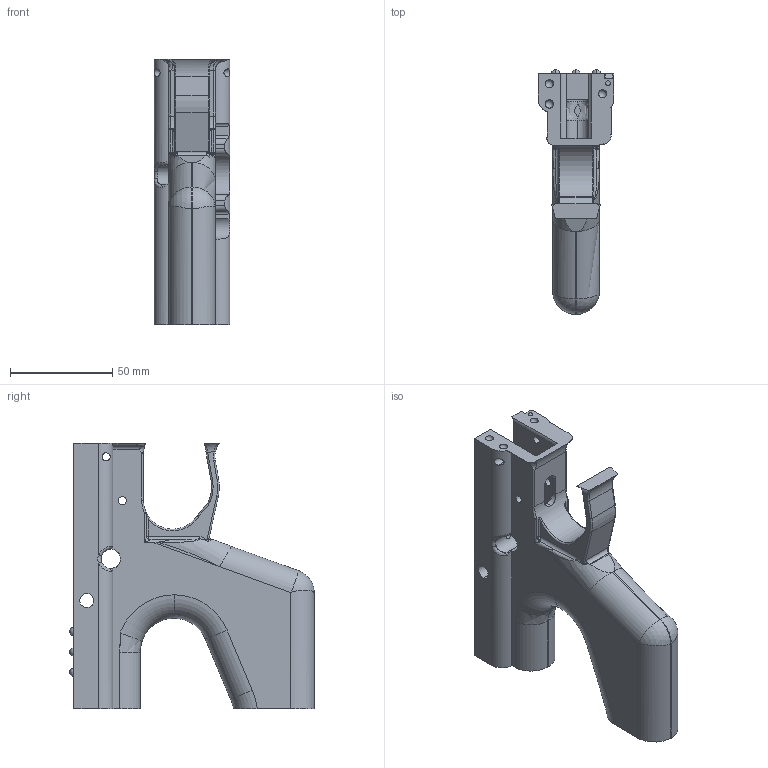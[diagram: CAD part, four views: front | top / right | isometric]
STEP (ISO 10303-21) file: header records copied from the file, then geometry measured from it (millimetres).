
FILE_DESCRIPTION (( 'STEP AP214' ), '1' );
FILE_NAME ('Unbuffered_Pistol_3.STEP', '2013-09-01T17:02:18', ( 'Asher' ), ( '' ), 'SwSTEP 2.0', 'SolidWorks 2013', '' );
FILE_SCHEMA (( 'AUTOMOTIVE_DESIGN' ));
Length unit declared in the file: millimetre
Products named in the file (1): Unbuffered_Pistol_3
Bounding box: 37.13 x 119.8 x 130 mm (x, y, z)
Volume: 202438.9 mm3; surface area: 40333.7 mm2
Topology: 1 solids, 1 shells, 255 faces, 719 edges, 444 vertices
Faces by surface type: cylinder 106, bspline 47, plane 45, torus 31, sphere 26
Entity records: 12213 total; most frequent: CARTESIAN_POINT 6182, ORIENTED_EDGE 1336, DIRECTION 1170, EDGE_CURVE 668, AXIS2_PLACEMENT_3D 470, VERTEX_POINT 425, EDGE_LOOP 285, CIRCLE 261
